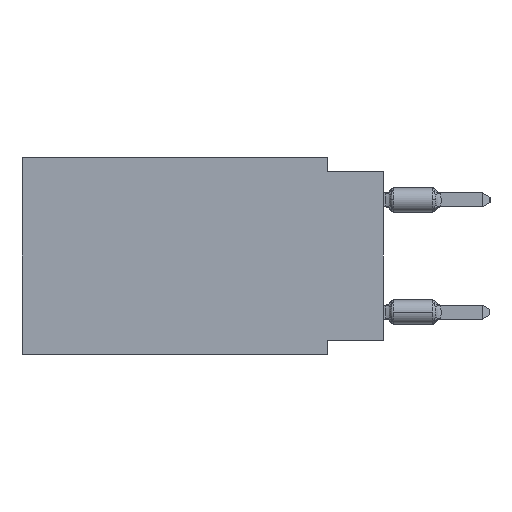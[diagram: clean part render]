
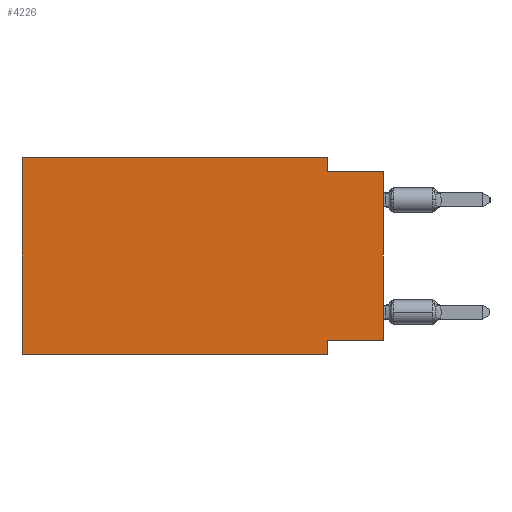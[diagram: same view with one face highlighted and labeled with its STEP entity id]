
A CAD part, left-side view. The second image highlights one B-rep face of the part: STEP entity #4226.
In plain terms, the highlighted planar face has unit normal (-1, 0, 0).
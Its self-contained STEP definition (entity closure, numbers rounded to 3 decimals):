
#32 = VECTOR ( 'NONE', #23673, 1000. ) ;
#198 = ORIENTED_EDGE ( 'NONE', *, *, #22635, .F. ) ;
#269 = DIRECTION ( 'NONE',  ( 0., -1., 0. ) ) ;
#583 = EDGE_CURVE ( 'NONE', #13926, #20059, #6297, .T. ) ;
#1445 = DIRECTION ( 'NONE',  ( 1., 0., 0. ) ) ;
#1582 = VERTEX_POINT ( 'NONE', #21647 ) ;
#1684 = LINE ( 'NONE', #12298, #9349 ) ;
#1997 = PLANE ( 'NONE',  #4203 ) ;
#2370 = CARTESIAN_POINT ( 'NONE',  ( 0., 16.383, -8.89 ) ) ;
#2485 = CARTESIAN_POINT ( 'NONE',  ( 0., 2.54, -8.255 ) ) ;
#3016 = VECTOR ( 'NONE', #269, 1000. ) ;
#3108 = LINE ( 'NONE', #26667, #15471 ) ;
#3968 = CARTESIAN_POINT ( 'NONE',  ( 0., 16.383, 0. ) ) ;
#4053 = LINE ( 'NONE', #6271, #32 ) ;
#4203 = AXIS2_PLACEMENT_3D ( 'NONE', #3968, #1445, #9947 ) ;
#4226 = ADVANCED_FACE ( 'NONE', ( #21182 ), #1997, .F. ) ;
#4365 = ORIENTED_EDGE ( 'NONE', *, *, #24844, .T. ) ;
#4814 = CARTESIAN_POINT ( 'NONE',  ( 0., 16.383, 0. ) ) ;
#4902 = EDGE_LOOP ( 'NONE', ( #4365, #10818, #6336, #16640, #25802, #10711, #198, #8899 ) ) ;
#5078 = VERTEX_POINT ( 'NONE', #27047 ) ;
#5086 = CARTESIAN_POINT ( 'NONE',  ( 0., 0., -8.255 ) ) ;
#5934 = CARTESIAN_POINT ( 'NONE',  ( 0., 2.54, -0.635 ) ) ;
#6271 = CARTESIAN_POINT ( 'NONE',  ( 0., 16.383, 0. ) ) ;
#6297 = LINE ( 'NONE', #10620, #10108 ) ;
#6336 = ORIENTED_EDGE ( 'NONE', *, *, #13395, .F. ) ;
#6416 = VERTEX_POINT ( 'NONE', #17198 ) ;
#7045 = DIRECTION ( 'NONE',  ( 0., -1., 0. ) ) ;
#8143 = VERTEX_POINT ( 'NONE', #5934 ) ;
#8516 = EDGE_CURVE ( 'NONE', #5078, #21789, #20215, .T. ) ;
#8899 = ORIENTED_EDGE ( 'NONE', *, *, #583, .F. ) ;
#9169 = VECTOR ( 'NONE', #9288, 1000. ) ;
#9288 = DIRECTION ( 'NONE',  ( 0., 0., 1. ) ) ;
#9349 = VECTOR ( 'NONE', #27497, 1000. ) ;
#9947 = DIRECTION ( 'NONE',  ( 0., 0., -1. ) ) ;
#10108 = VECTOR ( 'NONE', #21576, 1000. ) ;
#10620 = CARTESIAN_POINT ( 'NONE',  ( 0., 0., -8.255 ) ) ;
#10711 = ORIENTED_EDGE ( 'NONE', *, *, #15246, .T. ) ;
#10818 = ORIENTED_EDGE ( 'NONE', *, *, #17595, .F. ) ;
#10870 = EDGE_CURVE ( 'NONE', #6416, #5078, #4053, .T. ) ;
#11719 = DIRECTION ( 'NONE',  ( 0., 0., -1. ) ) ;
#11750 = DIRECTION ( 'NONE',  ( 0., 0., -1. ) ) ;
#12298 = CARTESIAN_POINT ( 'NONE',  ( 0., 0., -0.635 ) ) ;
#13395 = EDGE_CURVE ( 'NONE', #21789, #8143, #3108, .T. ) ;
#13926 = VERTEX_POINT ( 'NONE', #5086 ) ;
#14190 = VERTEX_POINT ( 'NONE', #14348 ) ;
#14348 = CARTESIAN_POINT ( 'NONE',  ( 0., 2.54, -8.89 ) ) ;
#15246 = EDGE_CURVE ( 'NONE', #6416, #14190, #19737, .T. ) ;
#15471 = VECTOR ( 'NONE', #11750, 1000. ) ;
#15803 = LINE ( 'NONE', #24659, #26293 ) ;
#16640 = ORIENTED_EDGE ( 'NONE', *, *, #8516, .F. ) ;
#17198 = CARTESIAN_POINT ( 'NONE',  ( 0., 16.383, -8.89 ) ) ;
#17595 = EDGE_CURVE ( 'NONE', #8143, #1582, #1684, .T. ) ;
#19708 = CARTESIAN_POINT ( 'NONE',  ( 0., 0., 0. ) ) ;
#19737 = LINE ( 'NONE', #2370, #3016 ) ;
#20059 = VERTEX_POINT ( 'NONE', #2485 ) ;
#20215 = LINE ( 'NONE', #4814, #20506 ) ;
#20505 = CARTESIAN_POINT ( 'NONE',  ( 0., 2.54, 0. ) ) ;
#20506 = VECTOR ( 'NONE', #7045, 1000. ) ;
#21182 = FACE_OUTER_BOUND ( 'NONE', #4902, .T. ) ;
#21576 = DIRECTION ( 'NONE',  ( 0., 1., 0. ) ) ;
#21647 = CARTESIAN_POINT ( 'NONE',  ( 0., 0., -0.635 ) ) ;
#21789 = VERTEX_POINT ( 'NONE', #20505 ) ;
#22214 = LINE ( 'NONE', #19708, #9169 ) ;
#22635 = EDGE_CURVE ( 'NONE', #20059, #14190, #15803, .T. ) ;
#23673 = DIRECTION ( 'NONE',  ( 0., 0., 1. ) ) ;
#24659 = CARTESIAN_POINT ( 'NONE',  ( 0., 2.54, -8.89 ) ) ;
#24844 = EDGE_CURVE ( 'NONE', #13926, #1582, #22214, .T. ) ;
#25802 = ORIENTED_EDGE ( 'NONE', *, *, #10870, .F. ) ;
#26293 = VECTOR ( 'NONE', #11719, 1000. ) ;
#26667 = CARTESIAN_POINT ( 'NONE',  ( 0., 2.54, 0. ) ) ;
#27047 = CARTESIAN_POINT ( 'NONE',  ( 0., 16.383, 0. ) ) ;
#27497 = DIRECTION ( 'NONE',  ( 0., -1., 0. ) ) ;
